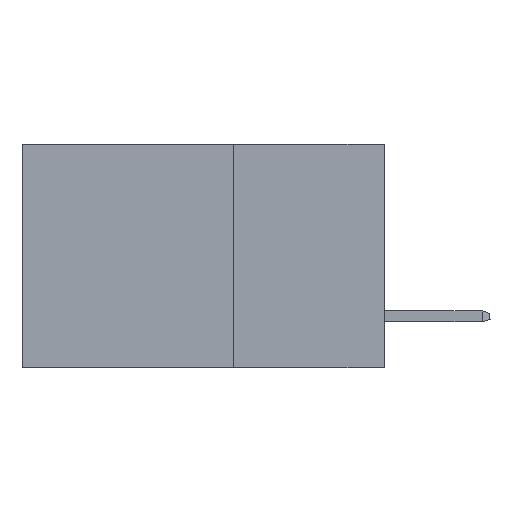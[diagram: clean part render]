
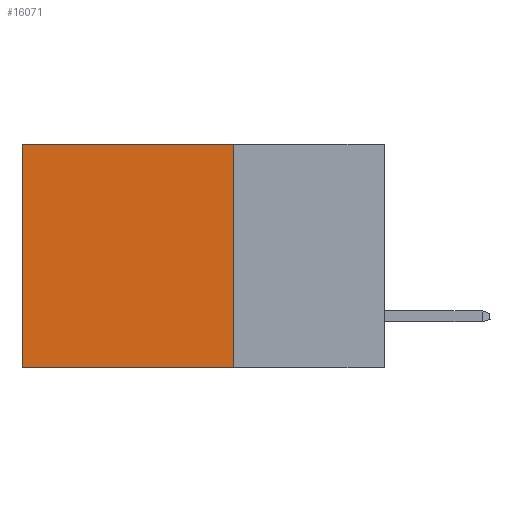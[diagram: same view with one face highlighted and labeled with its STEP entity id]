
A CAD part, left-side view. The second image highlights one B-rep face of the part: STEP entity #16071.
In plain terms, the highlighted planar face has unit normal (-1, 0, 0).
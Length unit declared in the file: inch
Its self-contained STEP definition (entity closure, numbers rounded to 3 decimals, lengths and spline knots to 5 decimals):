
#825 = CARTESIAN_POINT ( 'NONE',  ( 0.298, 0.25, -0.37 ) ) ;
#2050 = EDGE_LOOP ( 'NONE', ( #18663, #9895, #15608, #10881 ) ) ;
#2201 = DIRECTION ( 'NONE',  ( 0., 0., -1. ) ) ;
#2683 = VECTOR ( 'NONE', #14234, 39.37008 ) ;
#5038 = DIRECTION ( 'NONE',  ( 0., 1., 0. ) ) ;
#5402 = VERTEX_POINT ( 'NONE', #19758 ) ;
#6227 = CARTESIAN_POINT ( 'NONE',  ( 0.298, 0.25, 0. ) ) ;
#6923 = VERTEX_POINT ( 'NONE', #23949 ) ;
#7448 = CARTESIAN_POINT ( 'NONE',  ( 0.298, 0.6, 0. ) ) ;
#7753 = LINE ( 'NONE', #825, #14551 ) ;
#8685 = VERTEX_POINT ( 'NONE', #18357 ) ;
#9880 = CARTESIAN_POINT ( 'NONE',  ( 0.298, 0.25, 0. ) ) ;
#9895 = ORIENTED_EDGE ( 'NONE', *, *, #17912, .F. ) ;
#10078 = VECTOR ( 'NONE', #2201, 39.37008 ) ;
#10881 = ORIENTED_EDGE ( 'NONE', *, *, #11154, .T. ) ;
#11154 = EDGE_CURVE ( 'NONE', #16398, #5402, #25554, .T. ) ;
#11765 = FACE_OUTER_BOUND ( 'NONE', #2050, .T. ) ;
#12079 = DIRECTION ( 'NONE',  ( 0., 0., -1. ) ) ;
#13017 = EDGE_CURVE ( 'NONE', #16398, #8685, #24413, .T. ) ;
#13331 = CARTESIAN_POINT ( 'NONE',  ( 0.298, 0.25, 0. ) ) ;
#14234 = DIRECTION ( 'NONE',  ( 0., 1., 0. ) ) ;
#14301 = VECTOR ( 'NONE', #12079, 39.37008 ) ;
#14551 = VECTOR ( 'NONE', #5038, 39.37008 ) ;
#15608 = ORIENTED_EDGE ( 'NONE', *, *, #13017, .F. ) ;
#16071 = ADVANCED_FACE ( 'NONE', ( #11765 ), #23059, .F. ) ;
#16262 = AXIS2_PLACEMENT_3D ( 'NONE', #6227, #22871, #18692 ) ;
#16398 = VERTEX_POINT ( 'NONE', #13331 ) ;
#17912 = EDGE_CURVE ( 'NONE', #8685, #6923, #7753, .T. ) ;
#18357 = CARTESIAN_POINT ( 'NONE',  ( 0.298, 0.25, -0.37 ) ) ;
#18663 = ORIENTED_EDGE ( 'NONE', *, *, #24688, .T. ) ;
#18692 = DIRECTION ( 'NONE',  ( 0., 0., -1. ) ) ;
#19758 = CARTESIAN_POINT ( 'NONE',  ( 0.298, 0.6, 0. ) ) ;
#22871 = DIRECTION ( 'NONE',  ( 1., 0., 0. ) ) ;
#23059 = PLANE ( 'NONE',  #16262 ) ;
#23949 = CARTESIAN_POINT ( 'NONE',  ( 0.298, 0.6, -0.37 ) ) ;
#24413 = LINE ( 'NONE', #26822, #10078 ) ;
#24688 = EDGE_CURVE ( 'NONE', #5402, #6923, #26077, .T. ) ;
#25554 = LINE ( 'NONE', #9880, #2683 ) ;
#26077 = LINE ( 'NONE', #7448, #14301 ) ;
#26822 = CARTESIAN_POINT ( 'NONE',  ( 0.298, 0.25, 0. ) ) ;
